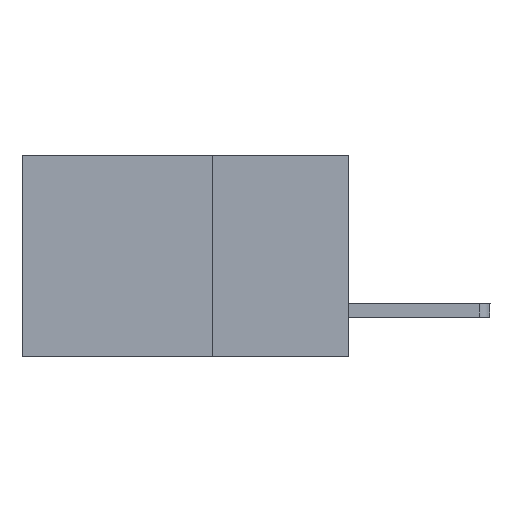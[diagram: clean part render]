
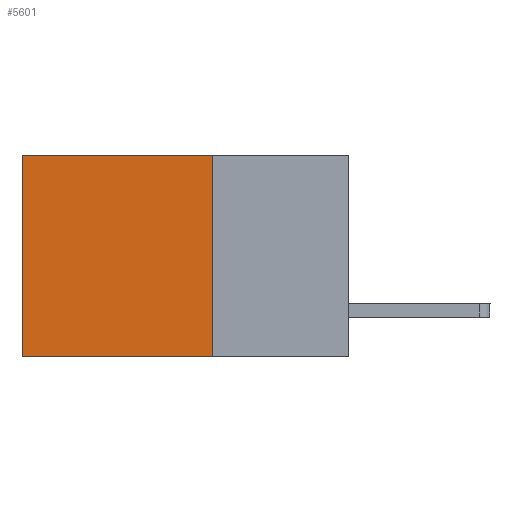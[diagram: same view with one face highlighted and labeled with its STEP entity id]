
A CAD part, left-side view. The second image highlights one B-rep face of the part: STEP entity #5601.
In plain terms, the highlighted planar face has unit normal (-1, 0, 0).
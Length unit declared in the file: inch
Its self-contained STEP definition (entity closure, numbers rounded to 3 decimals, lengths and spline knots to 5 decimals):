
#456 = CARTESIAN_POINT ( 'NONE',  ( 0.2615, 0.25, 0. ) ) ;
#1742 = DIRECTION ( 'NONE',  ( 0., 0., -1. ) ) ;
#2659 = CARTESIAN_POINT ( 'NONE',  ( 0.2615, 0.25, -0.37 ) ) ;
#2796 = ORIENTED_EDGE ( 'NONE', *, *, #7385, .T. ) ;
#3297 = VECTOR ( 'NONE', #6893, 39.37008 ) ;
#3329 = VECTOR ( 'NONE', #3431, 39.37008 ) ;
#3431 = DIRECTION ( 'NONE',  ( 0., 1., 0. ) ) ;
#3578 = DIRECTION ( 'NONE',  ( 0., 1., 0. ) ) ;
#3622 = LINE ( 'NONE', #8566, #6877 ) ;
#4136 = CARTESIAN_POINT ( 'NONE',  ( 0.2615, 0.25, -0.37 ) ) ;
#4260 = CARTESIAN_POINT ( 'NONE',  ( 0.2615, 0.25, -0.37 ) ) ;
#4443 = ORIENTED_EDGE ( 'NONE', *, *, #5101, .F. ) ;
#4585 = EDGE_CURVE ( 'NONE', #7707, #5050, #5267, .T. ) ;
#4740 = FACE_OUTER_BOUND ( 'NONE', #8897, .T. ) ;
#5050 = VERTEX_POINT ( 'NONE', #6240 ) ;
#5101 = EDGE_CURVE ( 'NONE', #5526, #6060, #7688, .T. ) ;
#5267 = LINE ( 'NONE', #8116, #7414 ) ;
#5328 = CARTESIAN_POINT ( 'NONE',  ( 0.2615, 0.6, 0. ) ) ;
#5492 = DIRECTION ( 'NONE',  ( 1., 0., 0. ) ) ;
#5526 = VERTEX_POINT ( 'NONE', #456 ) ;
#5558 = LINE ( 'NONE', #9016, #3329 ) ;
#5601 = ADVANCED_FACE ( 'NONE', ( #4740 ), #6186, .F. ) ;
#6060 = VERTEX_POINT ( 'NONE', #4260 ) ;
#6186 = PLANE ( 'NONE',  #8951 ) ;
#6240 = CARTESIAN_POINT ( 'NONE',  ( 0.2615, 0.6, -0.37 ) ) ;
#6877 = VECTOR ( 'NONE', #3578, 39.37008 ) ;
#6893 = DIRECTION ( 'NONE',  ( 0., 0., -1. ) ) ;
#7106 = EDGE_CURVE ( 'NONE', #6060, #5050, #3622, .T. ) ;
#7385 = EDGE_CURVE ( 'NONE', #5526, #7707, #5558, .T. ) ;
#7414 = VECTOR ( 'NONE', #1742, 39.37008 ) ;
#7424 = ORIENTED_EDGE ( 'NONE', *, *, #4585, .T. ) ;
#7688 = LINE ( 'NONE', #4136, #3297 ) ;
#7707 = VERTEX_POINT ( 'NONE', #5328 ) ;
#8116 = CARTESIAN_POINT ( 'NONE',  ( 0.2615, 0.6, -0.37 ) ) ;
#8341 = DIRECTION ( 'NONE',  ( 0., 0., -1. ) ) ;
#8566 = CARTESIAN_POINT ( 'NONE',  ( 0.2615, 0.25, -0.37 ) ) ;
#8647 = ORIENTED_EDGE ( 'NONE', *, *, #7106, .F. ) ;
#8897 = EDGE_LOOP ( 'NONE', ( #7424, #8647, #4443, #2796 ) ) ;
#8951 = AXIS2_PLACEMENT_3D ( 'NONE', #2659, #5492, #8341 ) ;
#9016 = CARTESIAN_POINT ( 'NONE',  ( 0.2615, 0.25, 0. ) ) ;
